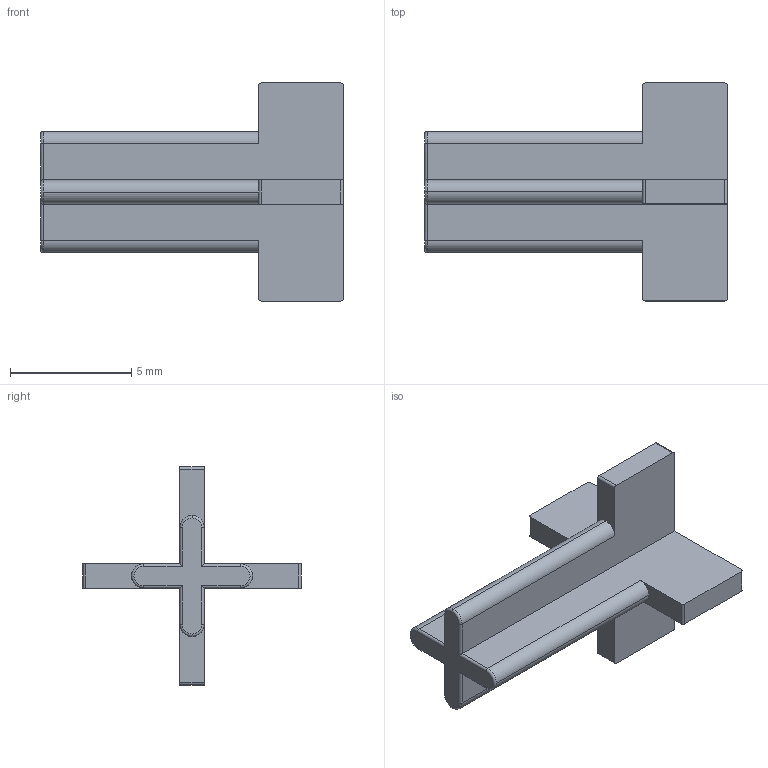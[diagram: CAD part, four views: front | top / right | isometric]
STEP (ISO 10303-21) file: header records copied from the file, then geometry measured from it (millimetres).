
FILE_DESCRIPTION (( 'STEP AP203' ), '1' );
FILE_NAME ('back_plate_gear.STEP', '2013-09-24T10:05:51', ( '' ), ( '' ), 'SwSTEP 2.0', 'SolidWorks 2012', '' );
FILE_SCHEMA (( 'CONFIG_CONTROL_DESIGN' ));
Length unit declared in the file: millimetre
Products named in the file (1): back_plate_gear
Bounding box: 12.5 x 9 x 9 mm (x, y, z)
Volume: 136.6 mm3; surface area: 323.4 mm2
Topology: 1 solids, 1 shells, 47 faces, 122 edges, 77 vertices
Faces by surface type: cylinder 24, plane 18, torus 5
Entity records: 1515 total; most frequent: DIRECTION 260, CARTESIAN_POINT 259, ORIENTED_EDGE 244, EDGE_CURVE 122, AXIS2_PLACEMENT_3D 94, VERTEX_POINT 77, LINE 72, VECTOR 72
